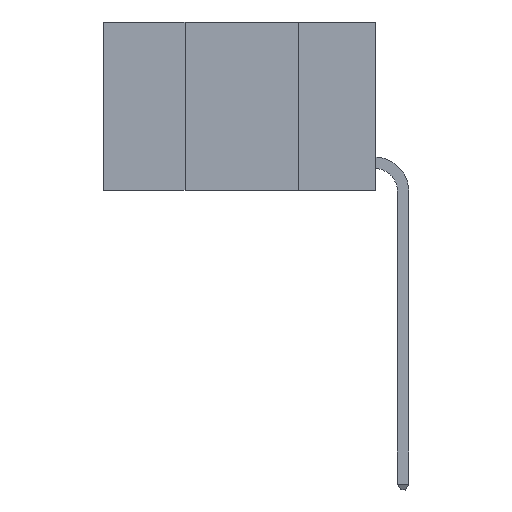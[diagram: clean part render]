
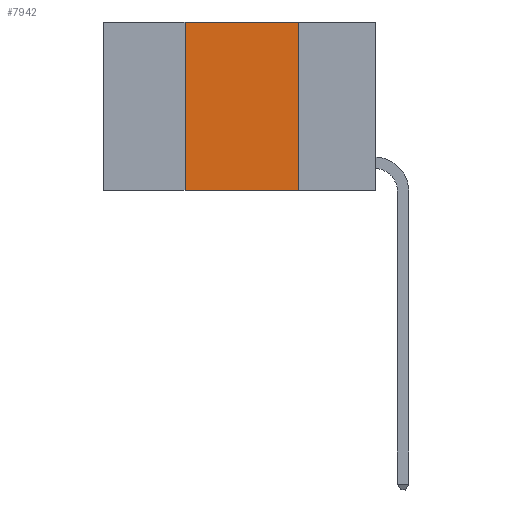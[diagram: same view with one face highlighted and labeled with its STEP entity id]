
A CAD part, left-side view. The second image highlights one B-rep face of the part: STEP entity #7942.
In plain terms, the highlighted planar face has unit normal (-1, 0, 0).
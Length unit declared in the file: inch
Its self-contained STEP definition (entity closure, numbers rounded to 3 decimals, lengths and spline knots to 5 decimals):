
#612 = FACE_OUTER_BOUND ( 'NONE', #15663, .T. ) ;
#759 = ORIENTED_EDGE ( 'NONE', *, *, #1520, .T. ) ;
#1165 = ORIENTED_EDGE ( 'NONE', *, *, #12229, .F. ) ;
#1283 = CARTESIAN_POINT ( 'NONE',  ( 0., 0.42, 0. ) ) ;
#1520 = EDGE_CURVE ( 'NONE', #10271, #13884, #13594, .T. ) ;
#1624 = CARTESIAN_POINT ( 'NONE',  ( 0., 0.17, 0. ) ) ;
#2886 = DIRECTION ( 'NONE',  ( 0., 0., 1. ) ) ;
#3022 = VERTEX_POINT ( 'NONE', #1624 ) ;
#3168 = CARTESIAN_POINT ( 'NONE',  ( 0., 0.42, -0.37 ) ) ;
#4658 = CARTESIAN_POINT ( 'NONE',  ( 0., 0.6, 0. ) ) ;
#4739 = ORIENTED_EDGE ( 'NONE', *, *, #15624, .F. ) ;
#5713 = DIRECTION ( 'NONE',  ( 0., 0., -1. ) ) ;
#6169 = AXIS2_PLACEMENT_3D ( 'NONE', #4658, #14766, #7288 ) ;
#6870 = CARTESIAN_POINT ( 'NONE',  ( 0., 0.6, 0. ) ) ;
#7004 = VECTOR ( 'NONE', #2886, 39.37008 ) ;
#7288 = DIRECTION ( 'NONE',  ( 0., 0., -1. ) ) ;
#7942 = ADVANCED_FACE ( 'NONE', ( #612 ), #9770, .F. ) ;
#9409 = LINE ( 'NONE', #13272, #15984 ) ;
#9770 = PLANE ( 'NONE',  #6169 ) ;
#10271 = VERTEX_POINT ( 'NONE', #3168 ) ;
#10290 = VECTOR ( 'NONE', #13727, 39.37008 ) ;
#10418 = CARTESIAN_POINT ( 'NONE',  ( 0., 0.17, -0.37 ) ) ;
#10727 = ORIENTED_EDGE ( 'NONE', *, *, #12823, .F. ) ;
#11008 = LINE ( 'NONE', #6870, #13936 ) ;
#11865 = CARTESIAN_POINT ( 'NONE',  ( 0., 0.42, 0. ) ) ;
#12229 = EDGE_CURVE ( 'NONE', #3022, #13884, #9409, .T. ) ;
#12823 = EDGE_CURVE ( 'NONE', #10271, #13876, #13266, .T. ) ;
#13266 = LINE ( 'NONE', #11865, #7004 ) ;
#13272 = CARTESIAN_POINT ( 'NONE',  ( 0., 0.17, 0. ) ) ;
#13594 = LINE ( 'NONE', #13840, #10290 ) ;
#13727 = DIRECTION ( 'NONE',  ( 0., -1., 0. ) ) ;
#13840 = CARTESIAN_POINT ( 'NONE',  ( 0., 0.6, -0.37 ) ) ;
#13876 = VERTEX_POINT ( 'NONE', #1283 ) ;
#13884 = VERTEX_POINT ( 'NONE', #10418 ) ;
#13936 = VECTOR ( 'NONE', #14353, 39.37008 ) ;
#14353 = DIRECTION ( 'NONE',  ( 0., -1., 0. ) ) ;
#14766 = DIRECTION ( 'NONE',  ( 1., 0., 0. ) ) ;
#15624 = EDGE_CURVE ( 'NONE', #13876, #3022, #11008, .T. ) ;
#15663 = EDGE_LOOP ( 'NONE', ( #1165, #4739, #10727, #759 ) ) ;
#15984 = VECTOR ( 'NONE', #5713, 39.37008 ) ;
